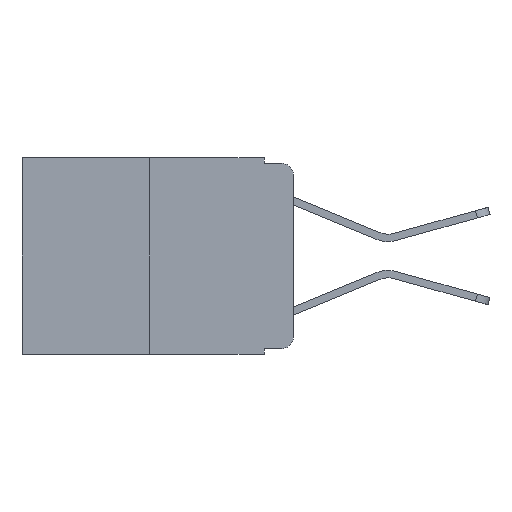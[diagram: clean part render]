
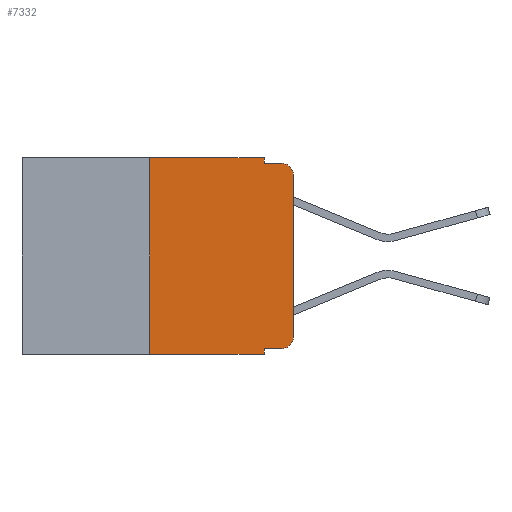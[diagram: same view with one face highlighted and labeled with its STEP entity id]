
A CAD part, left-side view. The second image highlights one B-rep face of the part: STEP entity #7332.
In plain terms, the highlighted planar face has unit normal (-1, 0, 0).
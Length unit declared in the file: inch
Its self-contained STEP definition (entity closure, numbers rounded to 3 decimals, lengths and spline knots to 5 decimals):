
#66 = CARTESIAN_POINT ( 'NONE',  ( 0., 0.02, -0.313 ) ) ;
#534 = LINE ( 'NONE', #10320, #16397 ) ;
#542 = CARTESIAN_POINT ( 'NONE',  ( 0., 0.25, 0. ) ) ;
#922 = EDGE_CURVE ( 'NONE', #17805, #2719, #534, .T. ) ;
#951 = LINE ( 'NONE', #3718, #6360 ) ;
#957 = PLANE ( 'NONE',  #11677 ) ;
#962 = CARTESIAN_POINT ( 'NONE',  ( 0., 0., -0.313 ) ) ;
#1045 = CARTESIAN_POINT ( 'NONE',  ( 0., 0.473, -0.343 ) ) ;
#1168 = VERTEX_POINT ( 'NONE', #11250 ) ;
#1534 = DIRECTION ( 'NONE',  ( 0., 0., -1. ) ) ;
#1649 = VECTOR ( 'NONE', #3914, 39.37008 ) ;
#2025 = CARTESIAN_POINT ( 'NONE',  ( 0., 0.02, -0.03 ) ) ;
#2181 = DIRECTION ( 'NONE',  ( 0., -1., 0. ) ) ;
#2341 = DIRECTION ( 'NONE',  ( 0., 0., -1. ) ) ;
#2499 = VECTOR ( 'NONE', #15759, 39.37008 ) ;
#2517 = CIRCLE ( 'NONE', #4593, 0.02 ) ;
#2719 = VERTEX_POINT ( 'NONE', #9084 ) ;
#2872 = VERTEX_POINT ( 'NONE', #15129 ) ;
#2924 = LINE ( 'NONE', #14148, #14691 ) ;
#3051 = CARTESIAN_POINT ( 'NONE',  ( 0., 0.051, 0. ) ) ;
#3280 = ORIENTED_EDGE ( 'NONE', *, *, #13379, .T. ) ;
#3718 = CARTESIAN_POINT ( 'NONE',  ( 0., 0.051, 0. ) ) ;
#3849 = EDGE_CURVE ( 'NONE', #2872, #12236, #8127, .T. ) ;
#3914 = DIRECTION ( 'NONE',  ( 0., -1., 0. ) ) ;
#3919 = EDGE_CURVE ( 'NONE', #6024, #2872, #2924, .T. ) ;
#4005 = FACE_OUTER_BOUND ( 'NONE', #8214, .T. ) ;
#4477 = CARTESIAN_POINT ( 'NONE',  ( 0., 0.25, 0. ) ) ;
#4593 = AXIS2_PLACEMENT_3D ( 'NONE', #2025, #8860, #14801 ) ;
#4675 = DIRECTION ( 'NONE',  ( 0., -1., 0. ) ) ;
#4939 = CARTESIAN_POINT ( 'NONE',  ( 0., 0.051, -0.333 ) ) ;
#5348 = CARTESIAN_POINT ( 'NONE',  ( 0., 0.25, -0.343 ) ) ;
#5451 = VECTOR ( 'NONE', #14138, 39.37008 ) ;
#5514 = LINE ( 'NONE', #15708, #5451 ) ;
#5881 = EDGE_CURVE ( 'NONE', #14592, #17805, #18310, .T. ) ;
#6024 = VERTEX_POINT ( 'NONE', #4939 ) ;
#6262 = ORIENTED_EDGE ( 'NONE', *, *, #7428, .T. ) ;
#6319 = VECTOR ( 'NONE', #16634, 39.37008 ) ;
#6360 = VECTOR ( 'NONE', #2341, 39.37008 ) ;
#6688 = DIRECTION ( 'NONE',  ( 0., 0., -1. ) ) ;
#6715 = CARTESIAN_POINT ( 'NONE',  ( 0., 0.051, -0.01 ) ) ;
#6801 = ORIENTED_EDGE ( 'NONE', *, *, #14826, .F. ) ;
#7101 = ORIENTED_EDGE ( 'NONE', *, *, #11407, .T. ) ;
#7303 = LINE ( 'NONE', #3051, #2499 ) ;
#7332 = ADVANCED_FACE ( 'NONE', ( #4005 ), #957, .F. ) ;
#7428 = EDGE_CURVE ( 'NONE', #14592, #13133, #8060, .T. ) ;
#7643 = VECTOR ( 'NONE', #17002, 39.37008 ) ;
#7724 = ORIENTED_EDGE ( 'NONE', *, *, #12111, .F. ) ;
#7877 = ORIENTED_EDGE ( 'NONE', *, *, #13817, .F. ) ;
#8060 = LINE ( 'NONE', #1045, #1649 ) ;
#8127 = CIRCLE ( 'NONE', #12337, 0.02 ) ;
#8214 = EDGE_LOOP ( 'NONE', ( #3280, #7101, #7724, #7877, #15964, #15300, #6262, #6801, #15770, #12049 ) ) ;
#8261 = DIRECTION ( 'NONE',  ( 1., 0., 0. ) ) ;
#8473 = DIRECTION ( 'NONE',  ( -1., 0., 0. ) ) ;
#8860 = DIRECTION ( 'NONE',  ( -1., 0., 0. ) ) ;
#9084 = CARTESIAN_POINT ( 'NONE',  ( 0., 0.051, 0. ) ) ;
#9620 = VERTEX_POINT ( 'NONE', #11759 ) ;
#10320 = CARTESIAN_POINT ( 'NONE',  ( 0., 0.473, 0. ) ) ;
#11143 = CARTESIAN_POINT ( 'NONE',  ( 0., 0., 0. ) ) ;
#11250 = CARTESIAN_POINT ( 'NONE',  ( 0., 0., -0.03 ) ) ;
#11407 = EDGE_CURVE ( 'NONE', #1168, #9620, #2517, .T. ) ;
#11677 = AXIS2_PLACEMENT_3D ( 'NONE', #16532, #8261, #6688 ) ;
#11759 = CARTESIAN_POINT ( 'NONE',  ( 0., 0.02, -0.01 ) ) ;
#11907 = VERTEX_POINT ( 'NONE', #6715 ) ;
#12049 = ORIENTED_EDGE ( 'NONE', *, *, #3849, .T. ) ;
#12111 = EDGE_CURVE ( 'NONE', #11907, #9620, #5514, .T. ) ;
#12236 = VERTEX_POINT ( 'NONE', #962 ) ;
#12263 = CARTESIAN_POINT ( 'NONE',  ( 0., 0.051, -0.343 ) ) ;
#12337 = AXIS2_PLACEMENT_3D ( 'NONE', #66, #8473, #1534 ) ;
#13133 = VERTEX_POINT ( 'NONE', #12263 ) ;
#13379 = EDGE_CURVE ( 'NONE', #12236, #1168, #18116, .T. ) ;
#13817 = EDGE_CURVE ( 'NONE', #2719, #11907, #7303, .T. ) ;
#14138 = DIRECTION ( 'NONE',  ( 0., -1., 0. ) ) ;
#14148 = CARTESIAN_POINT ( 'NONE',  ( 0., 0.051, -0.333 ) ) ;
#14592 = VERTEX_POINT ( 'NONE', #5348 ) ;
#14691 = VECTOR ( 'NONE', #4675, 39.37008 ) ;
#14801 = DIRECTION ( 'NONE',  ( 0., 0., -1. ) ) ;
#14826 = EDGE_CURVE ( 'NONE', #6024, #13133, #951, .T. ) ;
#15129 = CARTESIAN_POINT ( 'NONE',  ( 0., 0.02, -0.333 ) ) ;
#15300 = ORIENTED_EDGE ( 'NONE', *, *, #5881, .F. ) ;
#15708 = CARTESIAN_POINT ( 'NONE',  ( 0., 0.051, -0.01 ) ) ;
#15759 = DIRECTION ( 'NONE',  ( 0., 0., -1. ) ) ;
#15770 = ORIENTED_EDGE ( 'NONE', *, *, #3919, .T. ) ;
#15964 = ORIENTED_EDGE ( 'NONE', *, *, #922, .F. ) ;
#16397 = VECTOR ( 'NONE', #2181, 39.37008 ) ;
#16532 = CARTESIAN_POINT ( 'NONE',  ( 0., 0.473, 0. ) ) ;
#16634 = DIRECTION ( 'NONE',  ( 0., 0., 1. ) ) ;
#17002 = DIRECTION ( 'NONE',  ( 0., 0., 1. ) ) ;
#17805 = VERTEX_POINT ( 'NONE', #542 ) ;
#18116 = LINE ( 'NONE', #11143, #6319 ) ;
#18310 = LINE ( 'NONE', #4477, #7643 ) ;
